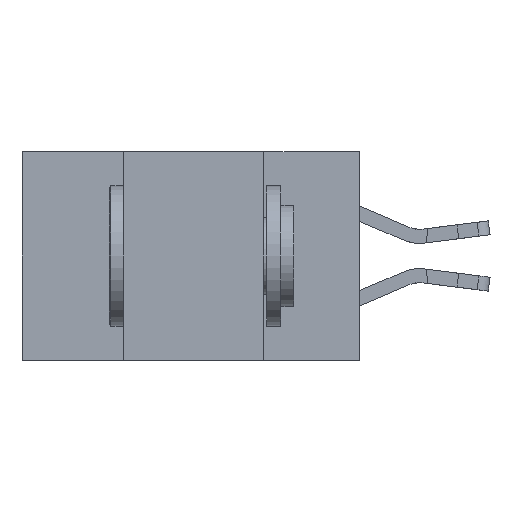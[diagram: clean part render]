
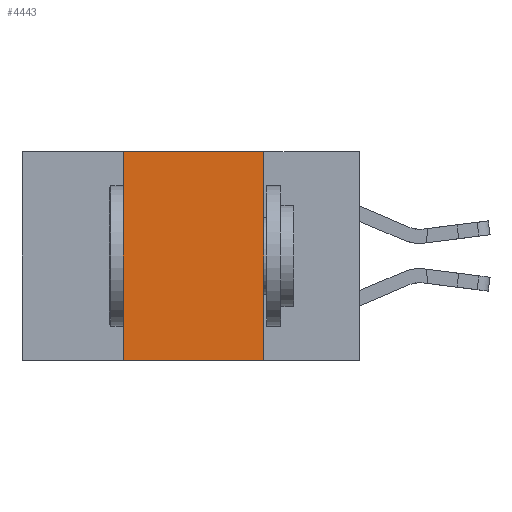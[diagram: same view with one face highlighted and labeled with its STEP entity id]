
A CAD part, left-side view. The second image highlights one B-rep face of the part: STEP entity #4443.
In plain terms, the highlighted planar face has unit normal (-1, 0, 0).
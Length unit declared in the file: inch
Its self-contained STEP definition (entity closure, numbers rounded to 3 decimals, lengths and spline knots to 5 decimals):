
#226 = ORIENTED_EDGE ( 'NONE', *, *, #20965, .F. ) ;
#784 = PLANE ( 'NONE',  #15232 ) ;
#1050 = LINE ( 'NONE', #12425, #21238 ) ;
#3033 = VERTEX_POINT ( 'NONE', #17517 ) ;
#3945 = DIRECTION ( 'NONE',  ( 0., -1., 0. ) ) ;
#4012 = CARTESIAN_POINT ( 'NONE',  ( 0., 0.17, -0.37 ) ) ;
#4443 = ADVANCED_FACE ( 'NONE', ( #10884 ), #784, .F. ) ;
#4867 = DIRECTION ( 'NONE',  ( 0., -1., 0. ) ) ;
#5917 = EDGE_CURVE ( 'NONE', #3033, #6813, #7733, .T. ) ;
#6577 = VERTEX_POINT ( 'NONE', #9578 ) ;
#6813 = VERTEX_POINT ( 'NONE', #4012 ) ;
#7733 = LINE ( 'NONE', #10396, #18161 ) ;
#8113 = VECTOR ( 'NONE', #4867, 39.37008 ) ;
#8393 = EDGE_LOOP ( 'NONE', ( #8582, #26861, #226, #12905 ) ) ;
#8582 = ORIENTED_EDGE ( 'NONE', *, *, #5917, .F. ) ;
#9578 = CARTESIAN_POINT ( 'NONE',  ( 0., 0.42, -0.37 ) ) ;
#10062 = VECTOR ( 'NONE', #11004, 39.37008 ) ;
#10396 = CARTESIAN_POINT ( 'NONE',  ( 0., 0.17, 0. ) ) ;
#10884 = FACE_OUTER_BOUND ( 'NONE', #8393, .T. ) ;
#11004 = DIRECTION ( 'NONE',  ( 0., 0., 1. ) ) ;
#11254 = DIRECTION ( 'NONE',  ( 1., 0., 0. ) ) ;
#12425 = CARTESIAN_POINT ( 'NONE',  ( 0., 0.6, 0. ) ) ;
#12438 = CARTESIAN_POINT ( 'NONE',  ( 0., 0.6, -0.37 ) ) ;
#12905 = ORIENTED_EDGE ( 'NONE', *, *, #21676, .T. ) ;
#13508 = DIRECTION ( 'NONE',  ( 0., 0., -1. ) ) ;
#14823 = VERTEX_POINT ( 'NONE', #26461 ) ;
#15232 = AXIS2_PLACEMENT_3D ( 'NONE', #23703, #11254, #13508 ) ;
#17517 = CARTESIAN_POINT ( 'NONE',  ( 0., 0.17, 0. ) ) ;
#18161 = VECTOR ( 'NONE', #24679, 39.37008 ) ;
#18852 = LINE ( 'NONE', #12438, #8113 ) ;
#19118 = CARTESIAN_POINT ( 'NONE',  ( 0., 0.42, 0. ) ) ;
#20965 = EDGE_CURVE ( 'NONE', #6577, #14823, #21795, .T. ) ;
#21238 = VECTOR ( 'NONE', #3945, 39.37008 ) ;
#21676 = EDGE_CURVE ( 'NONE', #6577, #6813, #18852, .T. ) ;
#21795 = LINE ( 'NONE', #19118, #10062 ) ;
#23703 = CARTESIAN_POINT ( 'NONE',  ( 0., 0.6, 0. ) ) ;
#24679 = DIRECTION ( 'NONE',  ( 0., 0., -1. ) ) ;
#25253 = EDGE_CURVE ( 'NONE', #14823, #3033, #1050, .T. ) ;
#26461 = CARTESIAN_POINT ( 'NONE',  ( 0., 0.42, 0. ) ) ;
#26861 = ORIENTED_EDGE ( 'NONE', *, *, #25253, .F. ) ;
